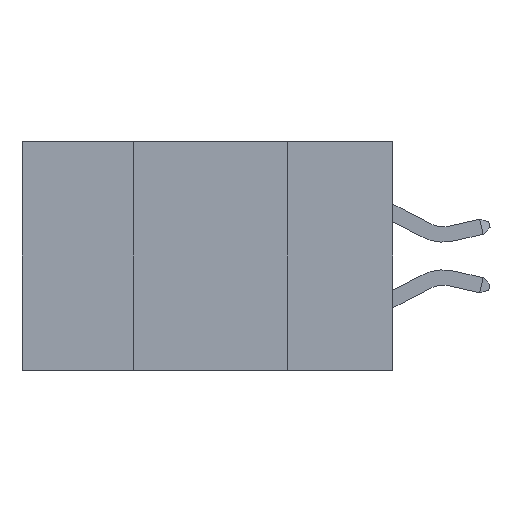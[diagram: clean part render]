
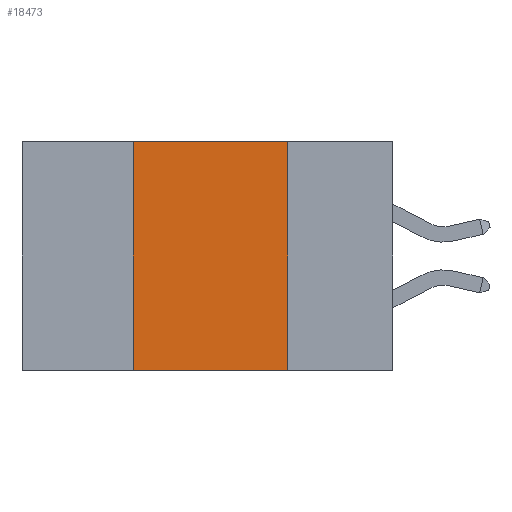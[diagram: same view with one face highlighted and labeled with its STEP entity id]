
A CAD part, left-side view. The second image highlights one B-rep face of the part: STEP entity #18473.
In plain terms, the highlighted planar face has unit normal (-1, 0, 0).
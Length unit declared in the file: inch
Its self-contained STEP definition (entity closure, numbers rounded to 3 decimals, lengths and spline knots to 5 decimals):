
#550 = ORIENTED_EDGE ( 'NONE', *, *, #8079, .F. ) ;
#1518 = CARTESIAN_POINT ( 'NONE',  ( 0., 0.17, 0. ) ) ;
#2018 = VERTEX_POINT ( 'NONE', #7096 ) ;
#2138 = LINE ( 'NONE', #6406, #13966 ) ;
#2445 = CARTESIAN_POINT ( 'NONE',  ( 0., 0.42, 0. ) ) ;
#4944 = VECTOR ( 'NONE', #5299, 39.37008 ) ;
#5299 = DIRECTION ( 'NONE',  ( 0., 0., 1. ) ) ;
#5415 = DIRECTION ( 'NONE',  ( 0., 0., -1. ) ) ;
#6406 = CARTESIAN_POINT ( 'NONE',  ( 0., 0.6, 0. ) ) ;
#6594 = DIRECTION ( 'NONE',  ( 0., -1., 0. ) ) ;
#6742 = PLANE ( 'NONE',  #11541 ) ;
#6876 = VERTEX_POINT ( 'NONE', #15051 ) ;
#7096 = CARTESIAN_POINT ( 'NONE',  ( 0., 0.17, 0. ) ) ;
#7545 = CARTESIAN_POINT ( 'NONE',  ( 0., 0.6, -0.37 ) ) ;
#7879 = ORIENTED_EDGE ( 'NONE', *, *, #10544, .F. ) ;
#8079 = EDGE_CURVE ( 'NONE', #2018, #6876, #17323, .T. ) ;
#8730 = VERTEX_POINT ( 'NONE', #13194 ) ;
#10410 = EDGE_CURVE ( 'NONE', #8730, #6876, #16404, .T. ) ;
#10501 = DIRECTION ( 'NONE',  ( 0., -1., 0. ) ) ;
#10544 = EDGE_CURVE ( 'NONE', #14191, #2018, #2138, .T. ) ;
#11413 = DIRECTION ( 'NONE',  ( 0., 0., -1. ) ) ;
#11541 = AXIS2_PLACEMENT_3D ( 'NONE', #12644, #12555, #5415 ) ;
#12400 = ORIENTED_EDGE ( 'NONE', *, *, #14268, .F. ) ;
#12555 = DIRECTION ( 'NONE',  ( 1., 0., 0. ) ) ;
#12644 = CARTESIAN_POINT ( 'NONE',  ( 0., 0.6, 0. ) ) ;
#13194 = CARTESIAN_POINT ( 'NONE',  ( 0., 0.42, -0.37 ) ) ;
#13966 = VECTOR ( 'NONE', #6594, 39.37008 ) ;
#14191 = VERTEX_POINT ( 'NONE', #2445 ) ;
#14268 = EDGE_CURVE ( 'NONE', #8730, #14191, #15205, .T. ) ;
#15051 = CARTESIAN_POINT ( 'NONE',  ( 0., 0.17, -0.37 ) ) ;
#15205 = LINE ( 'NONE', #18345, #4944 ) ;
#16404 = LINE ( 'NONE', #7545, #16933 ) ;
#16933 = VECTOR ( 'NONE', #10501, 39.37008 ) ;
#16938 = FACE_OUTER_BOUND ( 'NONE', #17666, .T. ) ;
#17323 = LINE ( 'NONE', #1518, #18461 ) ;
#17666 = EDGE_LOOP ( 'NONE', ( #550, #7879, #12400, #18420 ) ) ;
#18345 = CARTESIAN_POINT ( 'NONE',  ( 0., 0.42, 0. ) ) ;
#18420 = ORIENTED_EDGE ( 'NONE', *, *, #10410, .T. ) ;
#18461 = VECTOR ( 'NONE', #11413, 39.37008 ) ;
#18473 = ADVANCED_FACE ( 'NONE', ( #16938 ), #6742, .F. ) ;
